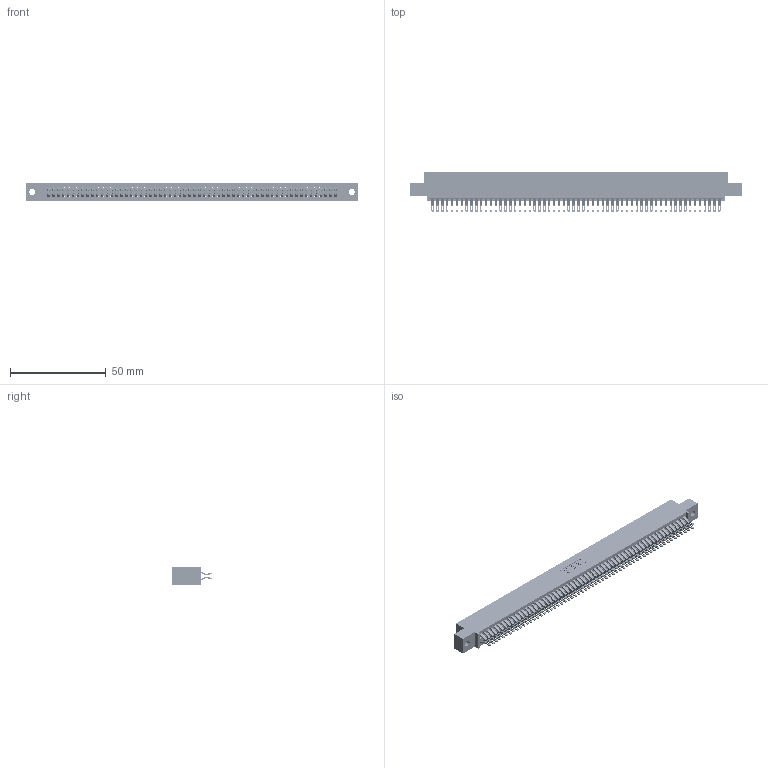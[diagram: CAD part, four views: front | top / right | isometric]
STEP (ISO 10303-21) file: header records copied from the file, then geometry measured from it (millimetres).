
FILE_DESCRIPTION (( 'STEP AP203' ), '1' );
FILE_NAME ('395-120-555-502.STEP', '2018-12-03T14:57:08', ( '' ), ( '' ), 'SwSTEP 2.0', 'SolidWorks 2016', '' );
FILE_SCHEMA (( 'CONFIG_CONTROL_DESIGN' ));
Length unit declared in the file: inch
Products named in the file (3): 345 Part_0.110 Offset - 0.128 Dia; 345-292-001_555 Tail; 395-120-555-502
Assembly tree (121 placements, depth 2):
  395-120-555-502
    345 Part_0.110 Offset - 0.128 Dia
    345-292-001_555 Tail  x120
Bounding box: 173.61 x 21.13 x 9.4 mm (x, y, z)
Volume: 17269.7 mm3; surface area: 26906.8 mm2
Topology: 121 solids, 121 shells, 6850 faces, 21593 edges, 14394 vertices
Faces by surface type: plane 3804, cylinder 3046
Entity records: 45115 total; most frequent: CARTESIAN_POINT 7582, ORIENTED_EDGE 7486, DIRECTION 6631, EDGE_CURVE 3743, VECTOR 3351, LINE 3351, VERTEX_POINT 2494, AXIS2_PLACEMENT_3D 1640
